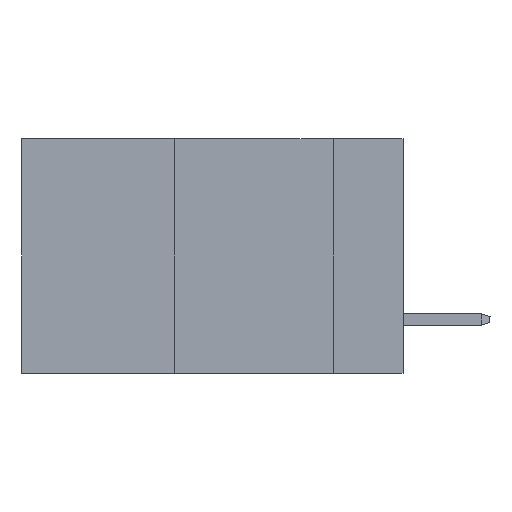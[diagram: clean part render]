
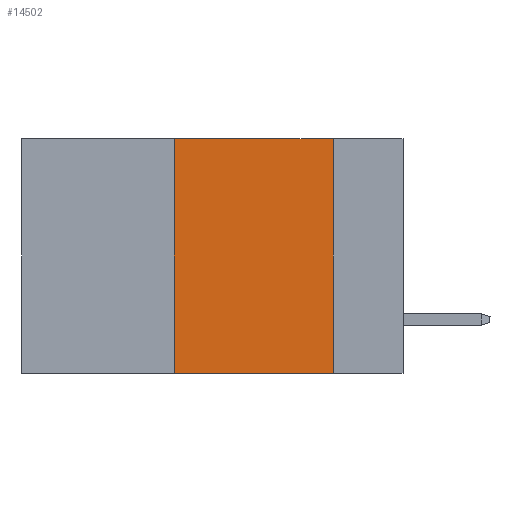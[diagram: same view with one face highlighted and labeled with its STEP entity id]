
A CAD part, left-side view. The second image highlights one B-rep face of the part: STEP entity #14502.
In plain terms, the highlighted planar face has unit normal (-1, 0, 0).
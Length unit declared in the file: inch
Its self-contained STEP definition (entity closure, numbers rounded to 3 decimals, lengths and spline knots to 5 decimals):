
#1315 = CARTESIAN_POINT ( 'NONE',  ( 0., 0.36, -0.37 ) ) ;
#1442 = CARTESIAN_POINT ( 'NONE',  ( 0., 0.6, -0.37 ) ) ;
#1475 = EDGE_LOOP ( 'NONE', ( #15195, #3956, #17689, #5642 ) ) ;
#1713 = VERTEX_POINT ( 'NONE', #9283 ) ;
#2015 = LINE ( 'NONE', #1442, #13999 ) ;
#2656 = EDGE_CURVE ( 'NONE', #20046, #1713, #6230, .T. ) ;
#3371 = CARTESIAN_POINT ( 'NONE',  ( 0., 0.36, 0. ) ) ;
#3575 = LINE ( 'NONE', #3371, #6898 ) ;
#3956 = ORIENTED_EDGE ( 'NONE', *, *, #2656, .F. ) ;
#5642 = ORIENTED_EDGE ( 'NONE', *, *, #6370, .T. ) ;
#5784 = CARTESIAN_POINT ( 'NONE',  ( 0., 0.11, 0. ) ) ;
#6230 = LINE ( 'NONE', #16081, #11213 ) ;
#6370 = EDGE_CURVE ( 'NONE', #14651, #12951, #2015, .T. ) ;
#6898 = VECTOR ( 'NONE', #13114, 39.37008 ) ;
#8417 = FACE_OUTER_BOUND ( 'NONE', #1475, .T. ) ;
#9283 = CARTESIAN_POINT ( 'NONE',  ( 0., 0.11, 0. ) ) ;
#9678 = DIRECTION ( 'NONE',  ( 0., -1., 0. ) ) ;
#10384 = VECTOR ( 'NONE', #13763, 39.37008 ) ;
#10923 = EDGE_CURVE ( 'NONE', #14651, #20046, #3575, .T. ) ;
#11213 = VECTOR ( 'NONE', #9678, 39.37008 ) ;
#12951 = VERTEX_POINT ( 'NONE', #14355 ) ;
#13114 = DIRECTION ( 'NONE',  ( 0., 0., 1. ) ) ;
#13763 = DIRECTION ( 'NONE',  ( 0., 0., -1. ) ) ;
#13871 = LINE ( 'NONE', #5784, #10384 ) ;
#13999 = VECTOR ( 'NONE', #17230, 39.37008 ) ;
#14355 = CARTESIAN_POINT ( 'NONE',  ( 0., 0.11, -0.37 ) ) ;
#14502 = ADVANCED_FACE ( 'NONE', ( #8417 ), #14738, .F. ) ;
#14651 = VERTEX_POINT ( 'NONE', #1315 ) ;
#14738 = PLANE ( 'NONE',  #18847 ) ;
#15195 = ORIENTED_EDGE ( 'NONE', *, *, #16278, .F. ) ;
#16081 = CARTESIAN_POINT ( 'NONE',  ( 0., 0.6, 0. ) ) ;
#16278 = EDGE_CURVE ( 'NONE', #1713, #12951, #13871, .T. ) ;
#16492 = CARTESIAN_POINT ( 'NONE',  ( 0., 0.6, 0. ) ) ;
#17230 = DIRECTION ( 'NONE',  ( 0., -1., 0. ) ) ;
#17689 = ORIENTED_EDGE ( 'NONE', *, *, #10923, .F. ) ;
#18164 = DIRECTION ( 'NONE',  ( 0., 0., -1. ) ) ;
#18847 = AXIS2_PLACEMENT_3D ( 'NONE', #16492, #19545, #18164 ) ;
#19545 = DIRECTION ( 'NONE',  ( 1., 0., 0. ) ) ;
#20046 = VERTEX_POINT ( 'NONE', #20209 ) ;
#20209 = CARTESIAN_POINT ( 'NONE',  ( 0., 0.36, 0. ) ) ;
